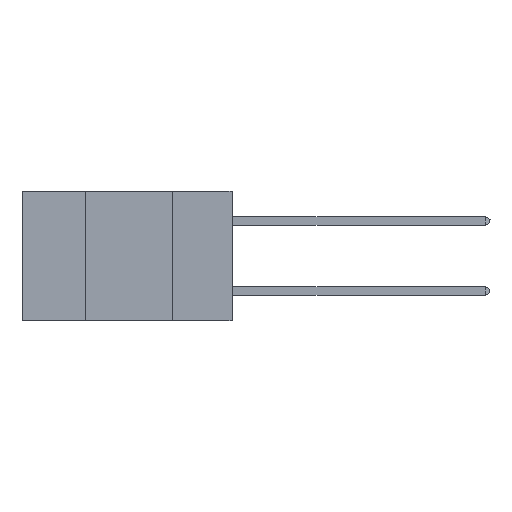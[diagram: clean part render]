
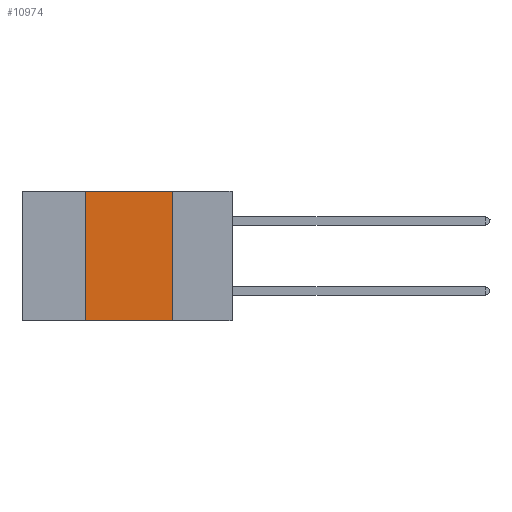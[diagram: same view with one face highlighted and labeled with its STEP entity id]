
A CAD part, left-side view. The second image highlights one B-rep face of the part: STEP entity #10974.
In plain terms, the highlighted planar face has unit normal (-1, 0, 0).
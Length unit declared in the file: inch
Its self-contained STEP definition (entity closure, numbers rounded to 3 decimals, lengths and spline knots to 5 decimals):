
#35 = DIRECTION ( 'NONE',  ( 1., 0., 0. ) ) ;
#729 = CARTESIAN_POINT ( 'NONE',  ( 0., 0.42, 0. ) ) ;
#1002 = DIRECTION ( 'NONE',  ( 0., -1., 0. ) ) ;
#1188 = PLANE ( 'NONE',  #8192 ) ;
#1572 = EDGE_CURVE ( 'NONE', #15696, #1674, #11001, .T. ) ;
#1674 = VERTEX_POINT ( 'NONE', #9673 ) ;
#3508 = EDGE_CURVE ( 'NONE', #14501, #1674, #15527, .T. ) ;
#4218 = CARTESIAN_POINT ( 'NONE',  ( 0., 0.6, 0. ) ) ;
#5804 = ORIENTED_EDGE ( 'NONE', *, *, #1572, .T. ) ;
#7128 = VECTOR ( 'NONE', #15637, 39.37008 ) ;
#7931 = CARTESIAN_POINT ( 'NONE',  ( 0., 0.17, 0. ) ) ;
#8098 = VECTOR ( 'NONE', #10535, 39.37008 ) ;
#8156 = CARTESIAN_POINT ( 'NONE',  ( 0., 0.6, -0.37 ) ) ;
#8192 = AXIS2_PLACEMENT_3D ( 'NONE', #4218, #35, #9854 ) ;
#8362 = ORIENTED_EDGE ( 'NONE', *, *, #17553, .F. ) ;
#8658 = ORIENTED_EDGE ( 'NONE', *, *, #11424, .F. ) ;
#9673 = CARTESIAN_POINT ( 'NONE',  ( 0., 0.17, -0.37 ) ) ;
#9854 = DIRECTION ( 'NONE',  ( 0., 0., -1. ) ) ;
#10054 = CARTESIAN_POINT ( 'NONE',  ( 0., 0.17, 0. ) ) ;
#10427 = VERTEX_POINT ( 'NONE', #729 ) ;
#10521 = VECTOR ( 'NONE', #1002, 39.37008 ) ;
#10535 = DIRECTION ( 'NONE',  ( 0., -1., 0. ) ) ;
#10974 = ADVANCED_FACE ( 'NONE', ( #11157 ), #1188, .F. ) ;
#11001 = LINE ( 'NONE', #8156, #10521 ) ;
#11157 = FACE_OUTER_BOUND ( 'NONE', #13687, .T. ) ;
#11424 = EDGE_CURVE ( 'NONE', #10427, #14501, #13108, .T. ) ;
#13108 = LINE ( 'NONE', #16075, #8098 ) ;
#13152 = ORIENTED_EDGE ( 'NONE', *, *, #3508, .F. ) ;
#13687 = EDGE_LOOP ( 'NONE', ( #13152, #8658, #8362, #5804 ) ) ;
#14501 = VERTEX_POINT ( 'NONE', #10054 ) ;
#14540 = LINE ( 'NONE', #15517, #7128 ) ;
#14894 = DIRECTION ( 'NONE',  ( 0., 0., -1. ) ) ;
#15517 = CARTESIAN_POINT ( 'NONE',  ( 0., 0.42, 0. ) ) ;
#15527 = LINE ( 'NONE', #7931, #17514 ) ;
#15637 = DIRECTION ( 'NONE',  ( 0., 0., 1. ) ) ;
#15696 = VERTEX_POINT ( 'NONE', #16003 ) ;
#16003 = CARTESIAN_POINT ( 'NONE',  ( 0., 0.42, -0.37 ) ) ;
#16075 = CARTESIAN_POINT ( 'NONE',  ( 0., 0.6, 0. ) ) ;
#17514 = VECTOR ( 'NONE', #14894, 39.37008 ) ;
#17553 = EDGE_CURVE ( 'NONE', #15696, #10427, #14540, .T. ) ;
